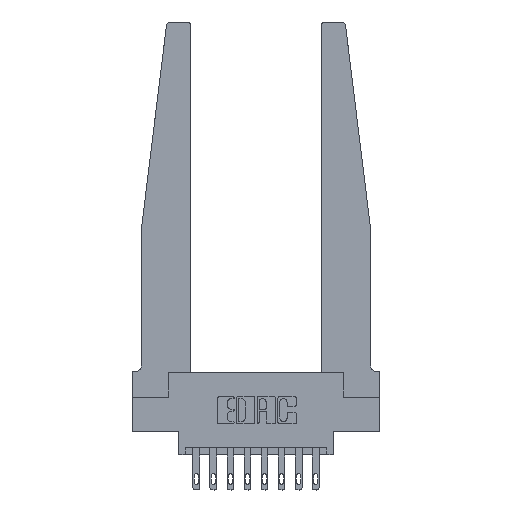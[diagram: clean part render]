
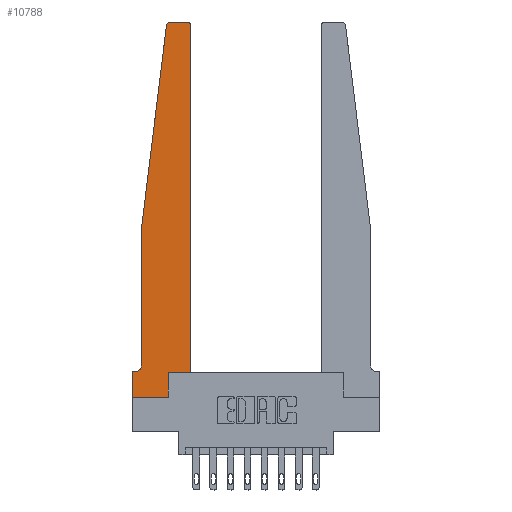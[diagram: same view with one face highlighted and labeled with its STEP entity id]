
A CAD part, top view. The second image highlights one B-rep face of the part: STEP entity #10788.
In plain terms, the highlighted planar face has unit normal (0, 0, 1).
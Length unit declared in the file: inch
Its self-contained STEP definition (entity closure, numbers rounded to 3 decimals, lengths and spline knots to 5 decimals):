
#42 = LINE ( 'NONE', #1184, #3287 ) ;
#99 = CARTESIAN_POINT ( 'NONE',  ( 0., 0., 0.37 ) ) ;
#427 = CARTESIAN_POINT ( 'NONE',  ( 0., 0., 0.37 ) ) ;
#472 = CARTESIAN_POINT ( 'NONE',  ( 0.2605, 0.18, 0.37 ) ) ;
#534 = CARTESIAN_POINT ( 'NONE',  ( 0.27653, 2.75, 0.37 ) ) ;
#617 = EDGE_CURVE ( 'NONE', #3224, #10082, #5151, .T. ) ;
#751 = CARTESIAN_POINT ( 'NONE',  ( 0.065, 1.25, 0.37 ) ) ;
#790 = CARTESIAN_POINT ( 'NONE',  ( 0.395, 2.75, 0.37 ) ) ;
#1015 = VECTOR ( 'NONE', #10693, 39.37008 ) ;
#1098 = DIRECTION ( 'NONE',  ( -1., 0., 0. ) ) ;
#1184 = CARTESIAN_POINT ( 'NONE',  ( 0.425, 0.18, 0.37 ) ) ;
#1206 = ORIENTED_EDGE ( 'NONE', *, *, #2413, .T. ) ;
#1212 = DIRECTION ( 'NONE',  ( 0., -1., 0. ) ) ;
#1265 = ORIENTED_EDGE ( 'NONE', *, *, #6974, .T. ) ;
#1348 = VERTEX_POINT ( 'NONE', #751 ) ;
#1548 = VECTOR ( 'NONE', #11195, 39.37008 ) ;
#1673 = VERTEX_POINT ( 'NONE', #13490 ) ;
#1687 = ORIENTED_EDGE ( 'NONE', *, *, #8563, .T. ) ;
#1740 = CIRCLE ( 'NONE', #11970, 0.03 ) ;
#2059 = DIRECTION ( 'NONE',  ( 1., 0., 0. ) ) ;
#2137 = DIRECTION ( 'NONE',  ( -0.122, -0.992, 0. ) ) ;
#2239 = LINE ( 'NONE', #6887, #8154 ) ;
#2383 = DIRECTION ( 'NONE',  ( 0., -1., 0. ) ) ;
#2413 = EDGE_CURVE ( 'NONE', #1348, #3224, #8238, .T. ) ;
#3043 = PLANE ( 'NONE',  #6435 ) ;
#3118 = ORIENTED_EDGE ( 'NONE', *, *, #12534, .T. ) ;
#3224 = VERTEX_POINT ( 'NONE', #13697 ) ;
#3253 = VERTEX_POINT ( 'NONE', #790 ) ;
#3287 = VECTOR ( 'NONE', #9363, 39.37008 ) ;
#3614 = EDGE_CURVE ( 'NONE', #7682, #13686, #12834, .T. ) ;
#3687 = ORIENTED_EDGE ( 'NONE', *, *, #3998, .T. ) ;
#3737 = CARTESIAN_POINT ( 'NONE',  ( 0.2605, 0.18, 0.37 ) ) ;
#3929 = LINE ( 'NONE', #427, #6562 ) ;
#3998 = EDGE_CURVE ( 'NONE', #9330, #1348, #5568, .T. ) ;
#4007 = ORIENTED_EDGE ( 'NONE', *, *, #14914, .T. ) ;
#4010 = CARTESIAN_POINT ( 'NONE',  ( 0.395, 2.72, 0.37 ) ) ;
#4173 = ORIENTED_EDGE ( 'NONE', *, *, #10102, .T. ) ;
#4174 = CIRCLE ( 'NONE', #6844, 0.03 ) ;
#4229 = EDGE_CURVE ( 'NONE', #13686, #10301, #3929, .T. ) ;
#4503 = CARTESIAN_POINT ( 'NONE',  ( 0., 0., 0.37 ) ) ;
#5017 = CARTESIAN_POINT ( 'NONE',  ( 0.015, 0.2375, 0.37 ) ) ;
#5076 = DIRECTION ( 'NONE',  ( 1., 0., 0. ) ) ;
#5101 = ORIENTED_EDGE ( 'NONE', *, *, #617, .T. ) ;
#5151 = CIRCLE ( 'NONE', #6382, 0.05 ) ;
#5230 = VERTEX_POINT ( 'NONE', #534 ) ;
#5568 = LINE ( 'NONE', #11591, #6315 ) ;
#6144 = EDGE_CURVE ( 'NONE', #11502, #3253, #4174, .T. ) ;
#6315 = VECTOR ( 'NONE', #2137, 39.37008 ) ;
#6382 = AXIS2_PLACEMENT_3D ( 'NONE', #5017, #9686, #13485 ) ;
#6435 = AXIS2_PLACEMENT_3D ( 'NONE', #7847, #12495, #2059 ) ;
#6545 = CARTESIAN_POINT ( 'NONE',  ( 0.425, 0.18, 0.37 ) ) ;
#6562 = VECTOR ( 'NONE', #5076, 39.37008 ) ;
#6577 = CARTESIAN_POINT ( 'NONE',  ( 0.24675, 2.72367, 0.37 ) ) ;
#6783 = LINE ( 'NONE', #11734, #7649 ) ;
#6844 = AXIS2_PLACEMENT_3D ( 'NONE', #4010, #9737, #10800 ) ;
#6887 = CARTESIAN_POINT ( 'NONE',  ( 0.065, 0.1875, 0.37 ) ) ;
#6974 = EDGE_CURVE ( 'NONE', #10301, #13034, #7317, .T. ) ;
#7317 = LINE ( 'NONE', #3737, #1015 ) ;
#7515 = CARTESIAN_POINT ( 'NONE',  ( 0.27653, 2.72, 0.37 ) ) ;
#7649 = VECTOR ( 'NONE', #9233, 39.37008 ) ;
#7678 = CARTESIAN_POINT ( 'NONE',  ( 0.425, 2.72, 0.37 ) ) ;
#7682 = VERTEX_POINT ( 'NONE', #9953 ) ;
#7847 = CARTESIAN_POINT ( 'NONE',  ( 0., 0.1875, 0.37 ) ) ;
#8154 = VECTOR ( 'NONE', #1098, 39.37008 ) ;
#8238 = LINE ( 'NONE', #8311, #15034 ) ;
#8311 = CARTESIAN_POINT ( 'NONE',  ( 0.065, 1.25, 0.37 ) ) ;
#8563 = EDGE_CURVE ( 'NONE', #3253, #5230, #6783, .T. ) ;
#9233 = DIRECTION ( 'NONE',  ( -1., 0., 0. ) ) ;
#9251 = ORIENTED_EDGE ( 'NONE', *, *, #4229, .T. ) ;
#9330 = VERTEX_POINT ( 'NONE', #6577 ) ;
#9363 = DIRECTION ( 'NONE',  ( 0., 1., 0. ) ) ;
#9512 = CARTESIAN_POINT ( 'NONE',  ( 0.015, 0.1875, 0.37 ) ) ;
#9686 = DIRECTION ( 'NONE',  ( 0., 0., -1. ) ) ;
#9737 = DIRECTION ( 'NONE',  ( 0., 0., 1. ) ) ;
#9953 = CARTESIAN_POINT ( 'NONE',  ( 0., 0.1875, 0.37 ) ) ;
#10082 = VERTEX_POINT ( 'NONE', #9512 ) ;
#10102 = EDGE_CURVE ( 'NONE', #1673, #11502, #42, .T. ) ;
#10261 = ORIENTED_EDGE ( 'NONE', *, *, #6144, .T. ) ;
#10301 = VERTEX_POINT ( 'NONE', #11440 ) ;
#10693 = DIRECTION ( 'NONE',  ( 0., 1., 0. ) ) ;
#10788 = ADVANCED_FACE ( 'NONE', ( #13499 ), #3043, .T. ) ;
#10800 = DIRECTION ( 'NONE',  ( 1., 0., 0. ) ) ;
#11195 = DIRECTION ( 'NONE',  ( 1., 0., 0. ) ) ;
#11199 = ORIENTED_EDGE ( 'NONE', *, *, #11688, .T. ) ;
#11392 = ORIENTED_EDGE ( 'NONE', *, *, #3614, .T. ) ;
#11440 = CARTESIAN_POINT ( 'NONE',  ( 0.2605, 0., 0.37 ) ) ;
#11502 = VERTEX_POINT ( 'NONE', #7678 ) ;
#11591 = CARTESIAN_POINT ( 'NONE',  ( 0.065, 1.25, 0.37 ) ) ;
#11688 = EDGE_CURVE ( 'NONE', #10082, #7682, #2239, .T. ) ;
#11734 = CARTESIAN_POINT ( 'NONE',  ( 0.25, 2.75, 0.37 ) ) ;
#11970 = AXIS2_PLACEMENT_3D ( 'NONE', #7515, #12158, #14663 ) ;
#12158 = DIRECTION ( 'NONE',  ( 0., 0., 1. ) ) ;
#12335 = LINE ( 'NONE', #6545, #1548 ) ;
#12495 = DIRECTION ( 'NONE',  ( 0., 0., 1. ) ) ;
#12534 = EDGE_CURVE ( 'NONE', #5230, #9330, #1740, .T. ) ;
#12834 = LINE ( 'NONE', #99, #13615 ) ;
#13034 = VERTEX_POINT ( 'NONE', #472 ) ;
#13485 = DIRECTION ( 'NONE',  ( -1., 0., 0. ) ) ;
#13490 = CARTESIAN_POINT ( 'NONE',  ( 0.425, 0.18, 0.37 ) ) ;
#13499 = FACE_OUTER_BOUND ( 'NONE', #14267, .T. ) ;
#13615 = VECTOR ( 'NONE', #2383, 39.37008 ) ;
#13686 = VERTEX_POINT ( 'NONE', #4503 ) ;
#13697 = CARTESIAN_POINT ( 'NONE',  ( 0.065, 0.2375, 0.37 ) ) ;
#14267 = EDGE_LOOP ( 'NONE', ( #1687, #3118, #3687, #1206, #5101, #11199, #11392, #9251, #1265, #4007, #4173, #10261 ) ) ;
#14663 = DIRECTION ( 'NONE',  ( 1., 0., 0. ) ) ;
#14914 = EDGE_CURVE ( 'NONE', #13034, #1673, #12335, .T. ) ;
#15034 = VECTOR ( 'NONE', #1212, 39.37008 ) ;
